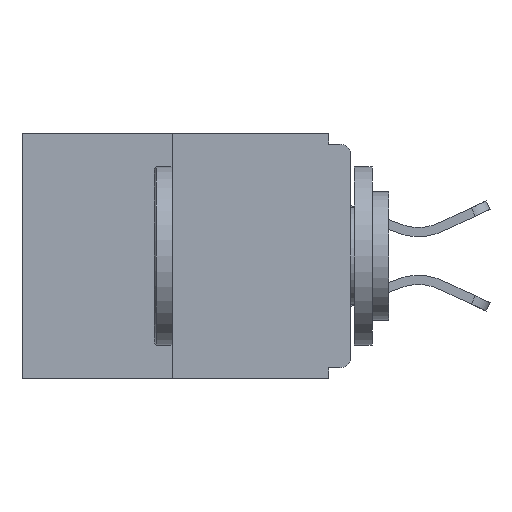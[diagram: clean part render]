
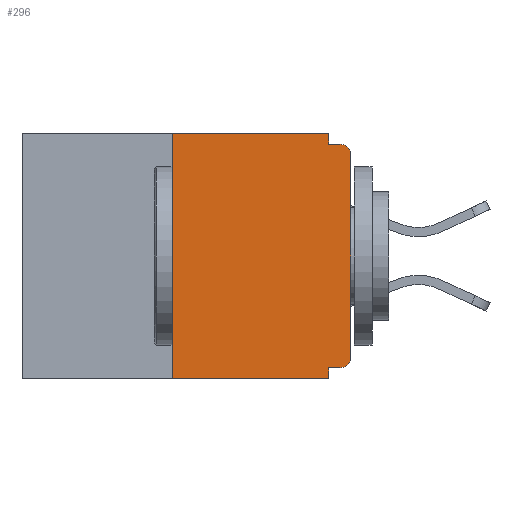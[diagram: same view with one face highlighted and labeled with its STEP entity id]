
A CAD part, left-side view. The second image highlights one B-rep face of the part: STEP entity #296.
In plain terms, the highlighted planar face has unit normal (-1, 0, 0).
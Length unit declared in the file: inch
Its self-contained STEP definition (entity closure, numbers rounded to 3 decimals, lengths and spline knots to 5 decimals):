
#245 = VERTEX_POINT ( 'NONE', #12186 ) ;
#296 = ADVANCED_FACE ( 'NONE', ( #5142 ), #12237, .F. ) ;
#311 = EDGE_CURVE ( 'NONE', #6114, #3584, #9980, .T. ) ;
#445 = VECTOR ( 'NONE', #10825, 39.37008 ) ;
#925 = CARTESIAN_POINT ( 'NONE',  ( 0., 0.46, -0.343 ) ) ;
#931 = VECTOR ( 'NONE', #5743, 39.37008 ) ;
#1256 = CARTESIAN_POINT ( 'NONE',  ( 0., 0.015, -0.328 ) ) ;
#1258 = DIRECTION ( 'NONE',  ( 0., 0., 1. ) ) ;
#1689 = CARTESIAN_POINT ( 'NONE',  ( 0., 0.46, 0. ) ) ;
#2154 = EDGE_CURVE ( 'NONE', #10950, #6114, #9130, .T. ) ;
#2247 = DIRECTION ( 'NONE',  ( 1., 0., 0. ) ) ;
#2627 = EDGE_CURVE ( 'NONE', #12782, #6562, #10296, .T. ) ;
#2702 = AXIS2_PLACEMENT_3D ( 'NONE', #9615, #2247, #10883 ) ;
#2908 = ORIENTED_EDGE ( 'NONE', *, *, #8831, .F. ) ;
#3261 = ORIENTED_EDGE ( 'NONE', *, *, #11898, .T. ) ;
#3584 = VERTEX_POINT ( 'NONE', #8533 ) ;
#3947 = DIRECTION ( 'NONE',  ( -1., 0., 0. ) ) ;
#4348 = ORIENTED_EDGE ( 'NONE', *, *, #14481, .T. ) ;
#4474 = DIRECTION ( 'NONE',  ( -1., 0., 0. ) ) ;
#4799 = ORIENTED_EDGE ( 'NONE', *, *, #10898, .F. ) ;
#5142 = FACE_OUTER_BOUND ( 'NONE', #15427, .T. ) ;
#5266 = VECTOR ( 'NONE', #9523, 39.37008 ) ;
#5363 = VERTEX_POINT ( 'NONE', #10083 ) ;
#5481 = CARTESIAN_POINT ( 'NONE',  ( 0., 0.031, -0.015 ) ) ;
#5743 = DIRECTION ( 'NONE',  ( 0., -1., 0. ) ) ;
#5801 = CARTESIAN_POINT ( 'NONE',  ( 0., 0.015, -0.015 ) ) ;
#5881 = CARTESIAN_POINT ( 'NONE',  ( 0., 0.015, -0.03 ) ) ;
#6114 = VERTEX_POINT ( 'NONE', #11527 ) ;
#6427 = CARTESIAN_POINT ( 'NONE',  ( 0., 0.031, 0. ) ) ;
#6562 = VERTEX_POINT ( 'NONE', #5481 ) ;
#6636 = LINE ( 'NONE', #7260, #11484 ) ;
#6700 = LINE ( 'NONE', #11939, #931 ) ;
#6963 = EDGE_CURVE ( 'NONE', #7660, #3584, #9929, .T. ) ;
#7029 = CIRCLE ( 'NONE', #10343, 0.015 ) ;
#7030 = VERTEX_POINT ( 'NONE', #5801 ) ;
#7260 = CARTESIAN_POINT ( 'NONE',  ( 0., 0.25, 0. ) ) ;
#7413 = AXIS2_PLACEMENT_3D ( 'NONE', #5881, #4474, #15666 ) ;
#7660 = VERTEX_POINT ( 'NONE', #10813 ) ;
#8533 = CARTESIAN_POINT ( 'NONE',  ( 0., 0.031, -0.343 ) ) ;
#8831 = EDGE_CURVE ( 'NONE', #5363, #12782, #15095, .T. ) ;
#9130 = LINE ( 'NONE', #15692, #5266 ) ;
#9486 = DIRECTION ( 'NONE',  ( 0., -1., 0. ) ) ;
#9523 = DIRECTION ( 'NONE',  ( 0., 1., 0. ) ) ;
#9615 = CARTESIAN_POINT ( 'NONE',  ( 0., 0.46, 0. ) ) ;
#9686 = VECTOR ( 'NONE', #13619, 39.37008 ) ;
#9929 = LINE ( 'NONE', #925, #15355 ) ;
#9980 = LINE ( 'NONE', #10983, #12901 ) ;
#10083 = CARTESIAN_POINT ( 'NONE',  ( 0., 0.25, 0. ) ) ;
#10241 = EDGE_CURVE ( 'NONE', #13732, #7030, #15069, .T. ) ;
#10284 = CARTESIAN_POINT ( 'NONE',  ( 0., 0., -0.03 ) ) ;
#10296 = LINE ( 'NONE', #11036, #445 ) ;
#10343 = AXIS2_PLACEMENT_3D ( 'NONE', #14024, #3947, #15141 ) ;
#10663 = LINE ( 'NONE', #14787, #9686 ) ;
#10733 = ORIENTED_EDGE ( 'NONE', *, *, #6963, .T. ) ;
#10813 = CARTESIAN_POINT ( 'NONE',  ( 0., 0.25, -0.343 ) ) ;
#10825 = DIRECTION ( 'NONE',  ( 0., 0., -1. ) ) ;
#10883 = DIRECTION ( 'NONE',  ( 0., 0., -1. ) ) ;
#10898 = EDGE_CURVE ( 'NONE', #6562, #7030, #6700, .T. ) ;
#10950 = VERTEX_POINT ( 'NONE', #1256 ) ;
#10983 = CARTESIAN_POINT ( 'NONE',  ( 0., 0.031, -0.343 ) ) ;
#11036 = CARTESIAN_POINT ( 'NONE',  ( 0., 0.031, 0. ) ) ;
#11484 = VECTOR ( 'NONE', #1258, 39.37008 ) ;
#11527 = CARTESIAN_POINT ( 'NONE',  ( 0., 0.031, -0.328 ) ) ;
#11898 = EDGE_CURVE ( 'NONE', #10950, #245, #7029, .T. ) ;
#11939 = CARTESIAN_POINT ( 'NONE',  ( 0., 0., -0.015 ) ) ;
#12186 = CARTESIAN_POINT ( 'NONE',  ( 0., 0., -0.313 ) ) ;
#12237 = PLANE ( 'NONE',  #2702 ) ;
#12782 = VERTEX_POINT ( 'NONE', #6427 ) ;
#12897 = EDGE_CURVE ( 'NONE', #7660, #5363, #6636, .T. ) ;
#12901 = VECTOR ( 'NONE', #13796, 39.37008 ) ;
#13229 = ORIENTED_EDGE ( 'NONE', *, *, #2154, .F. ) ;
#13619 = DIRECTION ( 'NONE',  ( 0., 0., 1. ) ) ;
#13732 = VERTEX_POINT ( 'NONE', #10284 ) ;
#13796 = DIRECTION ( 'NONE',  ( 0., 0., -1. ) ) ;
#13821 = ORIENTED_EDGE ( 'NONE', *, *, #2627, .F. ) ;
#14024 = CARTESIAN_POINT ( 'NONE',  ( 0., 0.015, -0.313 ) ) ;
#14481 = EDGE_CURVE ( 'NONE', #245, #13732, #10663, .T. ) ;
#14787 = CARTESIAN_POINT ( 'NONE',  ( 0., 0., 0. ) ) ;
#14795 = ORIENTED_EDGE ( 'NONE', *, *, #12897, .F. ) ;
#15018 = ORIENTED_EDGE ( 'NONE', *, *, #10241, .T. ) ;
#15069 = CIRCLE ( 'NONE', #7413, 0.015 ) ;
#15095 = LINE ( 'NONE', #1689, #15462 ) ;
#15125 = DIRECTION ( 'NONE',  ( 0., -1., 0. ) ) ;
#15141 = DIRECTION ( 'NONE',  ( 0., 0., -1. ) ) ;
#15355 = VECTOR ( 'NONE', #9486, 39.37008 ) ;
#15427 = EDGE_LOOP ( 'NONE', ( #2908, #14795, #10733, #15470, #13229, #3261, #4348, #15018, #4799, #13821 ) ) ;
#15462 = VECTOR ( 'NONE', #15125, 39.37008 ) ;
#15470 = ORIENTED_EDGE ( 'NONE', *, *, #311, .F. ) ;
#15666 = DIRECTION ( 'NONE',  ( 0., 0., -1. ) ) ;
#15692 = CARTESIAN_POINT ( 'NONE',  ( 0., 0., -0.328 ) ) ;
